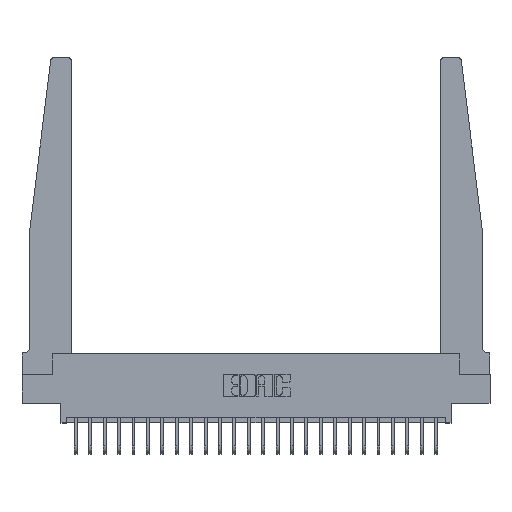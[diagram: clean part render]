
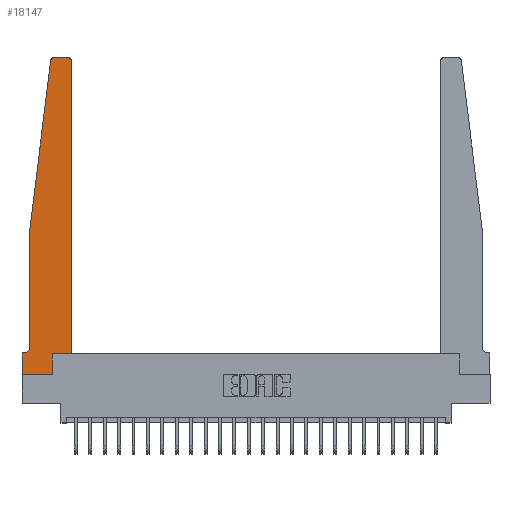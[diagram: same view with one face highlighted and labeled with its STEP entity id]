
A CAD part, top view. The second image highlights one B-rep face of the part: STEP entity #18147.
In plain terms, the highlighted planar face has unit normal (0, 0, 1).
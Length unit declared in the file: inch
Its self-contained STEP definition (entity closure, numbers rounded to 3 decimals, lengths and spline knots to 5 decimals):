
#1158 = LINE ( 'NONE', #19483, #16098 ) ;
#1614 = DIRECTION ( 'NONE',  ( 1., 0., 0. ) ) ;
#2028 = EDGE_CURVE ( 'NONE', #5352, #20674, #3296, .T. ) ;
#2557 = LINE ( 'NONE', #17037, #22932 ) ;
#2565 = VECTOR ( 'NONE', #19633, 39.37008 ) ;
#3296 = LINE ( 'NONE', #17529, #18965 ) ;
#3344 = LINE ( 'NONE', #5270, #20904 ) ;
#3874 = ORIENTED_EDGE ( 'NONE', *, *, #17164, .T. ) ;
#3893 = AXIS2_PLACEMENT_3D ( 'NONE', #17710, #8634, #5046 ) ;
#3933 = CARTESIAN_POINT ( 'NONE',  ( 0.015, 0.1875, 0.37 ) ) ;
#4521 = CARTESIAN_POINT ( 'NONE',  ( 0.25, 2.75, 0.37 ) ) ;
#4858 = CARTESIAN_POINT ( 'NONE',  ( 0.24675, 2.72367, 0.37 ) ) ;
#5046 = DIRECTION ( 'NONE',  ( 1., 0., 0. ) ) ;
#5200 = CARTESIAN_POINT ( 'NONE',  ( 0.395, 2.75, 0.37 ) ) ;
#5270 = CARTESIAN_POINT ( 'NONE',  ( 0.425, 0.18, 0.37 ) ) ;
#5352 = VERTEX_POINT ( 'NONE', #4858 ) ;
#5648 = CARTESIAN_POINT ( 'NONE',  ( 0.425, 0.18, 0.37 ) ) ;
#5649 = LINE ( 'NONE', #20141, #16894 ) ;
#6442 = CARTESIAN_POINT ( 'NONE',  ( 0.2605, 0.18, 0.37 ) ) ;
#6570 = DIRECTION ( 'NONE',  ( 0., 0., 1. ) ) ;
#6585 = VERTEX_POINT ( 'NONE', #6442 ) ;
#6613 = CIRCLE ( 'NONE', #8150, 0.03 ) ;
#6956 = CARTESIAN_POINT ( 'NONE',  ( 0.065, 1.25, 0.37 ) ) ;
#7016 = VERTEX_POINT ( 'NONE', #5648 ) ;
#7115 = CARTESIAN_POINT ( 'NONE',  ( 0., 0., 0.37 ) ) ;
#7419 = VERTEX_POINT ( 'NONE', #20236 ) ;
#7468 = ORIENTED_EDGE ( 'NONE', *, *, #14714, .T. ) ;
#7496 = VECTOR ( 'NONE', #17316, 39.37008 ) ;
#7979 = DIRECTION ( 'NONE',  ( -1., 0., 0. ) ) ;
#8150 = AXIS2_PLACEMENT_3D ( 'NONE', #10736, #6570, #1614 ) ;
#8235 = ORIENTED_EDGE ( 'NONE', *, *, #21379, .T. ) ;
#8496 = DIRECTION ( 'NONE',  ( 0., 1., 0. ) ) ;
#8512 = DIRECTION ( 'NONE',  ( 1., 0., 0. ) ) ;
#8634 = DIRECTION ( 'NONE',  ( 0., 0., 1. ) ) ;
#8772 = EDGE_CURVE ( 'NONE', #21248, #20628, #16955, .T. ) ;
#8936 = VERTEX_POINT ( 'NONE', #10847 ) ;
#9716 = EDGE_CURVE ( 'NONE', #6585, #7016, #3344, .T. ) ;
#9890 = VERTEX_POINT ( 'NONE', #3933 ) ;
#9999 = CIRCLE ( 'NONE', #23376, 0.05 ) ;
#10242 = DIRECTION ( 'NONE',  ( 0., -1., 0. ) ) ;
#10448 = ORIENTED_EDGE ( 'NONE', *, *, #11031, .T. ) ;
#10527 = CARTESIAN_POINT ( 'NONE',  ( 0.2605, 0., 0.37 ) ) ;
#10572 = ORIENTED_EDGE ( 'NONE', *, *, #8772, .T. ) ;
#10736 = CARTESIAN_POINT ( 'NONE',  ( 0.27653, 2.72, 0.37 ) ) ;
#10847 = CARTESIAN_POINT ( 'NONE',  ( 0., 0.1875, 0.37 ) ) ;
#10902 = LINE ( 'NONE', #14121, #21311 ) ;
#11031 = EDGE_CURVE ( 'NONE', #18524, #6585, #10902, .T. ) ;
#11070 = EDGE_CURVE ( 'NONE', #20674, #11437, #18073, .T. ) ;
#11437 = VERTEX_POINT ( 'NONE', #22977 ) ;
#11502 = DIRECTION ( 'NONE',  ( 0., 0., 1. ) ) ;
#11659 = EDGE_LOOP ( 'NONE', ( #10572, #21445, #16842, #15413, #3874, #7468, #8235, #16672, #10448, #20916, #17922, #17232 ) ) ;
#11710 = CARTESIAN_POINT ( 'NONE',  ( 0.065, 1.25, 0.37 ) ) ;
#12221 = FACE_OUTER_BOUND ( 'NONE', #11659, .T. ) ;
#13393 = DIRECTION ( 'NONE',  ( 0., 0., -1. ) ) ;
#14121 = CARTESIAN_POINT ( 'NONE',  ( 0.2605, 0.18, 0.37 ) ) ;
#14714 = EDGE_CURVE ( 'NONE', #9890, #8936, #2557, .T. ) ;
#14952 = AXIS2_PLACEMENT_3D ( 'NONE', #22895, #11502, #18804 ) ;
#15413 = ORIENTED_EDGE ( 'NONE', *, *, #11070, .T. ) ;
#15733 = CIRCLE ( 'NONE', #14952, 0.03 ) ;
#16098 = VECTOR ( 'NONE', #8496, 39.37008 ) ;
#16202 = LINE ( 'NONE', #7115, #17698 ) ;
#16672 = ORIENTED_EDGE ( 'NONE', *, *, #20239, .T. ) ;
#16842 = ORIENTED_EDGE ( 'NONE', *, *, #2028, .T. ) ;
#16894 = VECTOR ( 'NONE', #23639, 39.37008 ) ;
#16942 = EDGE_CURVE ( 'NONE', #7419, #21248, #15733, .T. ) ;
#16955 = LINE ( 'NONE', #4521, #7496 ) ;
#16961 = CARTESIAN_POINT ( 'NONE',  ( 0.015, 0.2375, 0.37 ) ) ;
#17037 = CARTESIAN_POINT ( 'NONE',  ( 0.065, 0.1875, 0.37 ) ) ;
#17164 = EDGE_CURVE ( 'NONE', #11437, #9890, #9999, .T. ) ;
#17232 = ORIENTED_EDGE ( 'NONE', *, *, #16942, .T. ) ;
#17316 = DIRECTION ( 'NONE',  ( -1., 0., 0. ) ) ;
#17529 = CARTESIAN_POINT ( 'NONE',  ( 0.065, 1.25, 0.37 ) ) ;
#17698 = VECTOR ( 'NONE', #10242, 39.37008 ) ;
#17710 = CARTESIAN_POINT ( 'NONE',  ( 0., 0.1875, 0.37 ) ) ;
#17922 = ORIENTED_EDGE ( 'NONE', *, *, #18616, .T. ) ;
#18073 = LINE ( 'NONE', #6956, #2565 ) ;
#18147 = ADVANCED_FACE ( 'NONE', ( #12221 ), #19516, .T. ) ;
#18524 = VERTEX_POINT ( 'NONE', #10527 ) ;
#18616 = EDGE_CURVE ( 'NONE', #7016, #7419, #1158, .T. ) ;
#18804 = DIRECTION ( 'NONE',  ( 1., 0., 0. ) ) ;
#18965 = VECTOR ( 'NONE', #19336, 39.37008 ) ;
#19336 = DIRECTION ( 'NONE',  ( -0.122, -0.992, 0. ) ) ;
#19483 = CARTESIAN_POINT ( 'NONE',  ( 0.425, 0.18, 0.37 ) ) ;
#19516 = PLANE ( 'NONE',  #3893 ) ;
#19633 = DIRECTION ( 'NONE',  ( 0., -1., 0. ) ) ;
#20141 = CARTESIAN_POINT ( 'NONE',  ( 0., 0., 0.37 ) ) ;
#20236 = CARTESIAN_POINT ( 'NONE',  ( 0.425, 2.72, 0.37 ) ) ;
#20239 = EDGE_CURVE ( 'NONE', #22324, #18524, #5649, .T. ) ;
#20628 = VERTEX_POINT ( 'NONE', #21686 ) ;
#20674 = VERTEX_POINT ( 'NONE', #11710 ) ;
#20816 = DIRECTION ( 'NONE',  ( -1., 0., 0. ) ) ;
#20886 = EDGE_CURVE ( 'NONE', #20628, #5352, #6613, .T. ) ;
#20904 = VECTOR ( 'NONE', #8512, 39.37008 ) ;
#20916 = ORIENTED_EDGE ( 'NONE', *, *, #9716, .T. ) ;
#21248 = VERTEX_POINT ( 'NONE', #5200 ) ;
#21309 = DIRECTION ( 'NONE',  ( 0., 1., 0. ) ) ;
#21311 = VECTOR ( 'NONE', #21309, 39.37008 ) ;
#21379 = EDGE_CURVE ( 'NONE', #8936, #22324, #16202, .T. ) ;
#21445 = ORIENTED_EDGE ( 'NONE', *, *, #20886, .T. ) ;
#21686 = CARTESIAN_POINT ( 'NONE',  ( 0.27653, 2.75, 0.37 ) ) ;
#22324 = VERTEX_POINT ( 'NONE', #22369 ) ;
#22369 = CARTESIAN_POINT ( 'NONE',  ( 0., 0., 0.37 ) ) ;
#22895 = CARTESIAN_POINT ( 'NONE',  ( 0.395, 2.72, 0.37 ) ) ;
#22932 = VECTOR ( 'NONE', #7979, 39.37008 ) ;
#22977 = CARTESIAN_POINT ( 'NONE',  ( 0.065, 0.2375, 0.37 ) ) ;
#23376 = AXIS2_PLACEMENT_3D ( 'NONE', #16961, #13393, #20816 ) ;
#23639 = DIRECTION ( 'NONE',  ( 1., 0., 0. ) ) ;
